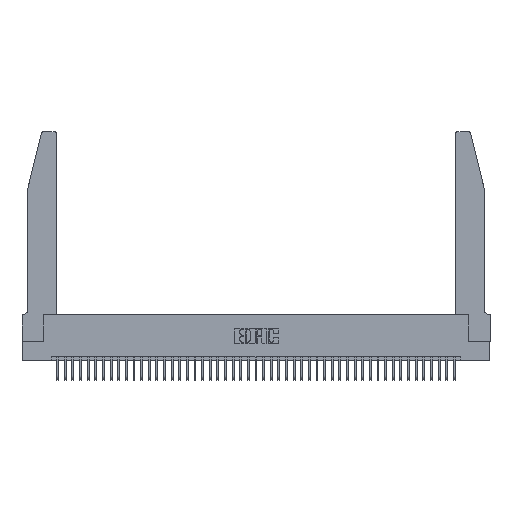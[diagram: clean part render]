
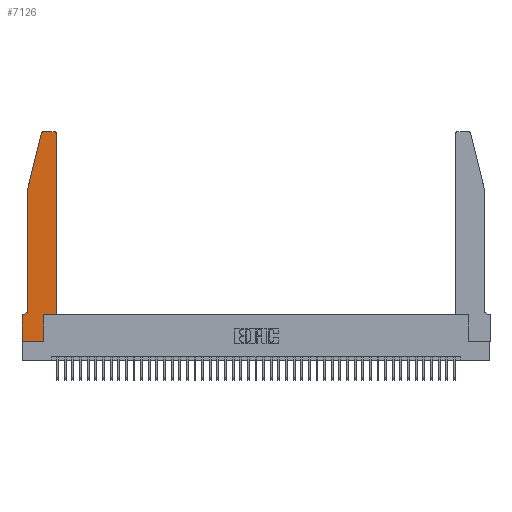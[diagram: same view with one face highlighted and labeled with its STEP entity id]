
A CAD part, top view. The second image highlights one B-rep face of the part: STEP entity #7126.
In plain terms, the highlighted planar face has unit normal (0, 0, 1).
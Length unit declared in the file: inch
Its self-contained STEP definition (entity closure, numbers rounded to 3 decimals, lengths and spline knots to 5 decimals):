
#551 = DIRECTION ( 'NONE',  ( 1., 0., 0. ) ) ;
#751 = CIRCLE ( 'NONE', #44399, 0.03 ) ;
#832 = DIRECTION ( 'NONE',  ( 0., 0., 1. ) ) ;
#1119 = DIRECTION ( 'NONE',  ( -1., 0., 0. ) ) ;
#1594 = CARTESIAN_POINT ( 'NONE',  ( 0.4205, 2.75, 0.37 ) ) ;
#2319 = VERTEX_POINT ( 'NONE', #5526 ) ;
#2425 = CARTESIAN_POINT ( 'NONE',  ( 0.25487, 2.72718, 0.37 ) ) ;
#2660 = EDGE_LOOP ( 'NONE', ( #5662, #16923, #15361, #11507, #5244, #17420, #10760, #4268, #17632, #34049, #19947, #25283 ) ) ;
#3515 = DIRECTION ( 'NONE',  ( 1., 0., 0. ) ) ;
#3814 = LINE ( 'NONE', #9856, #6070 ) ;
#4051 = DIRECTION ( 'NONE',  ( -1., 0., 0. ) ) ;
#4268 = ORIENTED_EDGE ( 'NONE', *, *, #33819, .T. ) ;
#4704 = CARTESIAN_POINT ( 'NONE',  ( 0.0755, 0.35, 0.37 ) ) ;
#5244 = ORIENTED_EDGE ( 'NONE', *, *, #19041, .T. ) ;
#5526 = CARTESIAN_POINT ( 'NONE',  ( 0.284, 2.75, 0.37 ) ) ;
#5662 = ORIENTED_EDGE ( 'NONE', *, *, #8509, .T. ) ;
#6070 = VECTOR ( 'NONE', #21735, 39.37008 ) ;
#6360 = CARTESIAN_POINT ( 'NONE',  ( 0.0755, 2., 0.37 ) ) ;
#6538 = CARTESIAN_POINT ( 'NONE',  ( 0.0755, 2., 0.37 ) ) ;
#7126 = ADVANCED_FACE ( 'NONE', ( #24190 ), #25680, .T. ) ;
#8088 = LINE ( 'NONE', #21225, #18243 ) ;
#8256 = VECTOR ( 'NONE', #37655, 39.37008 ) ;
#8509 = EDGE_CURVE ( 'NONE', #12754, #2319, #23151, .T. ) ;
#8526 = CARTESIAN_POINT ( 'NONE',  ( 0., 0., 0.37 ) ) ;
#9856 = CARTESIAN_POINT ( 'NONE',  ( 0.4505, 0.35, 0.37 ) ) ;
#10760 = ORIENTED_EDGE ( 'NONE', *, *, #17343, .T. ) ;
#11244 = CARTESIAN_POINT ( 'NONE',  ( 0.4505, 2.72, 0.37 ) ) ;
#11507 = ORIENTED_EDGE ( 'NONE', *, *, #16656, .T. ) ;
#11568 = CARTESIAN_POINT ( 'NONE',  ( 0.2605, 2.75, 0.37 ) ) ;
#12624 = AXIS2_PLACEMENT_3D ( 'NONE', #44757, #44581, #1119 ) ;
#12669 = CARTESIAN_POINT ( 'NONE',  ( 0.2865, 0.35, 0.37 ) ) ;
#12688 = CIRCLE ( 'NONE', #12624, 0.07 ) ;
#12754 = VERTEX_POINT ( 'NONE', #1594 ) ;
#13176 = CARTESIAN_POINT ( 'NONE',  ( 0.0755, 0.42, 0.37 ) ) ;
#13427 = LINE ( 'NONE', #39944, #29176 ) ;
#13697 = DIRECTION ( 'NONE',  ( -0.239, -0.971, 0. ) ) ;
#14430 = VECTOR ( 'NONE', #33927, 39.37008 ) ;
#15289 = EDGE_CURVE ( 'NONE', #22982, #42638, #20288, .T. ) ;
#15361 = ORIENTED_EDGE ( 'NONE', *, *, #27538, .T. ) ;
#15650 = VERTEX_POINT ( 'NONE', #28360 ) ;
#16030 = DIRECTION ( 'NONE',  ( 1., 0., 0. ) ) ;
#16603 = CIRCLE ( 'NONE', #35917, 0.03 ) ;
#16656 = EDGE_CURVE ( 'NONE', #29638, #23390, #33106, .T. ) ;
#16923 = ORIENTED_EDGE ( 'NONE', *, *, #34667, .T. ) ;
#17343 = EDGE_CURVE ( 'NONE', #42638, #15650, #32503, .T. ) ;
#17362 = VECTOR ( 'NONE', #19998, 39.37008 ) ;
#17420 = ORIENTED_EDGE ( 'NONE', *, *, #15289, .T. ) ;
#17632 = ORIENTED_EDGE ( 'NONE', *, *, #28648, .T. ) ;
#17908 = VECTOR ( 'NONE', #13697, 39.37008 ) ;
#18243 = VECTOR ( 'NONE', #24411, 39.37008 ) ;
#18268 = VERTEX_POINT ( 'NONE', #36898 ) ;
#18478 = CARTESIAN_POINT ( 'NONE',  ( 0.284, 2.72, 0.37 ) ) ;
#19041 = EDGE_CURVE ( 'NONE', #23390, #22982, #12688, .T. ) ;
#19279 = DIRECTION ( 'NONE',  ( -1., 0., 0. ) ) ;
#19947 = ORIENTED_EDGE ( 'NONE', *, *, #27802, .T. ) ;
#19957 = CARTESIAN_POINT ( 'NONE',  ( 0.4205, 2.72, 0.37 ) ) ;
#19998 = DIRECTION ( 'NONE',  ( 0., -1., 0. ) ) ;
#20099 = CARTESIAN_POINT ( 'NONE',  ( 0.2865, 0., 0.37 ) ) ;
#20288 = LINE ( 'NONE', #4704, #40541 ) ;
#21225 = CARTESIAN_POINT ( 'NONE',  ( 0., 0., 0.37 ) ) ;
#21735 = DIRECTION ( 'NONE',  ( 1., 0., 0. ) ) ;
#22982 = VERTEX_POINT ( 'NONE', #27887 ) ;
#23151 = LINE ( 'NONE', #11568, #32229 ) ;
#23390 = VERTEX_POINT ( 'NONE', #13176 ) ;
#24190 = FACE_OUTER_BOUND ( 'NONE', #2660, .T. ) ;
#24411 = DIRECTION ( 'NONE',  ( 1., 0., 0. ) ) ;
#24624 = LINE ( 'NONE', #12669, #14430 ) ;
#25283 = ORIENTED_EDGE ( 'NONE', *, *, #34236, .T. ) ;
#25295 = DIRECTION ( 'NONE',  ( 0., 1., 0. ) ) ;
#25680 = PLANE ( 'NONE',  #30073 ) ;
#26431 = VERTEX_POINT ( 'NONE', #11244 ) ;
#27538 = EDGE_CURVE ( 'NONE', #29565, #29638, #37042, .T. ) ;
#27802 = EDGE_CURVE ( 'NONE', #18268, #26431, #13427, .T. ) ;
#27887 = CARTESIAN_POINT ( 'NONE',  ( 0.0055, 0.35, 0.37 ) ) ;
#28360 = CARTESIAN_POINT ( 'NONE',  ( 0., 0., 0.37 ) ) ;
#28648 = EDGE_CURVE ( 'NONE', #43405, #44080, #24624, .T. ) ;
#29176 = VECTOR ( 'NONE', #25295, 39.37008 ) ;
#29565 = VERTEX_POINT ( 'NONE', #2425 ) ;
#29638 = VERTEX_POINT ( 'NONE', #6538 ) ;
#30073 = AXIS2_PLACEMENT_3D ( 'NONE', #45281, #41441, #3515 ) ;
#30896 = CARTESIAN_POINT ( 'NONE',  ( 0.0755, 2., 0.37 ) ) ;
#32229 = VECTOR ( 'NONE', #4051, 39.37008 ) ;
#32503 = LINE ( 'NONE', #8526, #8256 ) ;
#33106 = LINE ( 'NONE', #30896, #17362 ) ;
#33184 = EDGE_CURVE ( 'NONE', #44080, #18268, #3814, .T. ) ;
#33819 = EDGE_CURVE ( 'NONE', #15650, #43405, #8088, .T. ) ;
#33927 = DIRECTION ( 'NONE',  ( 0., 1., 0. ) ) ;
#34049 = ORIENTED_EDGE ( 'NONE', *, *, #33184, .T. ) ;
#34236 = EDGE_CURVE ( 'NONE', #26431, #12754, #16603, .T. ) ;
#34667 = EDGE_CURVE ( 'NONE', #2319, #29565, #751, .T. ) ;
#35917 = AXIS2_PLACEMENT_3D ( 'NONE', #19957, #37431, #16030 ) ;
#36898 = CARTESIAN_POINT ( 'NONE',  ( 0.4505, 0.35, 0.37 ) ) ;
#37042 = LINE ( 'NONE', #6360, #17908 ) ;
#37431 = DIRECTION ( 'NONE',  ( 0., 0., 1. ) ) ;
#37655 = DIRECTION ( 'NONE',  ( 0., -1., 0. ) ) ;
#39944 = CARTESIAN_POINT ( 'NONE',  ( 0.4505, 0.35, 0.37 ) ) ;
#40541 = VECTOR ( 'NONE', #19279, 39.37008 ) ;
#41441 = DIRECTION ( 'NONE',  ( 0., 0., 1. ) ) ;
#42638 = VERTEX_POINT ( 'NONE', #43456 ) ;
#43405 = VERTEX_POINT ( 'NONE', #20099 ) ;
#43456 = CARTESIAN_POINT ( 'NONE',  ( 0., 0.35, 0.37 ) ) ;
#44080 = VERTEX_POINT ( 'NONE', #45248 ) ;
#44399 = AXIS2_PLACEMENT_3D ( 'NONE', #18478, #832, #551 ) ;
#44581 = DIRECTION ( 'NONE',  ( 0., 0., -1. ) ) ;
#44757 = CARTESIAN_POINT ( 'NONE',  ( 0.0055, 0.42, 0.37 ) ) ;
#45248 = CARTESIAN_POINT ( 'NONE',  ( 0.2865, 0.35, 0.37 ) ) ;
#45281 = CARTESIAN_POINT ( 'NONE',  ( 0., 0.35, 0.37 ) ) ;
